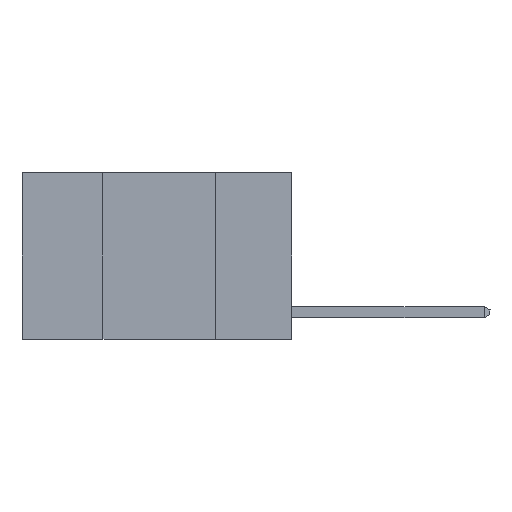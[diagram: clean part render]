
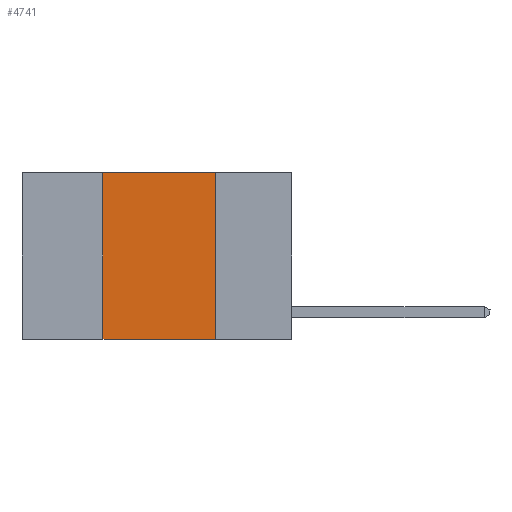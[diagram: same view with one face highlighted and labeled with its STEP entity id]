
A CAD part, left-side view. The second image highlights one B-rep face of the part: STEP entity #4741.
In plain terms, the highlighted planar face has unit normal (-1, 0, 0).
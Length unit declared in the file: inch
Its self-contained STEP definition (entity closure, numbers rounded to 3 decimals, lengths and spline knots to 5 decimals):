
#99 = FACE_OUTER_BOUND ( 'NONE', #6273, .T. ) ;
#701 = LINE ( 'NONE', #2503, #13827 ) ;
#1141 = VERTEX_POINT ( 'NONE', #3644 ) ;
#2503 = CARTESIAN_POINT ( 'NONE',  ( 0., 0.17, 0. ) ) ;
#2911 = DIRECTION ( 'NONE',  ( 1., 0., 0. ) ) ;
#3143 = ORIENTED_EDGE ( 'NONE', *, *, #4018, .F. ) ;
#3644 = CARTESIAN_POINT ( 'NONE',  ( 0., 0.17, -0.37 ) ) ;
#4018 = EDGE_CURVE ( 'NONE', #9808, #6234, #17129, .T. ) ;
#4741 = ADVANCED_FACE ( 'NONE', ( #99 ), #13741, .F. ) ;
#5187 = DIRECTION ( 'NONE',  ( 0., -1., 0. ) ) ;
#5517 = DIRECTION ( 'NONE',  ( 0., 0., -1. ) ) ;
#5796 = CARTESIAN_POINT ( 'NONE',  ( 0., 0.6, -0.37 ) ) ;
#5877 = ORIENTED_EDGE ( 'NONE', *, *, #19534, .T. ) ;
#6234 = VERTEX_POINT ( 'NONE', #14365 ) ;
#6273 = EDGE_LOOP ( 'NONE', ( #17300, #3143, #19536, #5877 ) ) ;
#7920 = CARTESIAN_POINT ( 'NONE',  ( 0., 0.42, 0. ) ) ;
#8238 = VECTOR ( 'NONE', #18033, 39.37008 ) ;
#8359 = EDGE_CURVE ( 'NONE', #10522, #9808, #13824, .T. ) ;
#8941 = DIRECTION ( 'NONE',  ( 0., 0., -1. ) ) ;
#9808 = VERTEX_POINT ( 'NONE', #14621 ) ;
#10199 = LINE ( 'NONE', #5796, #8238 ) ;
#10522 = VERTEX_POINT ( 'NONE', #15298 ) ;
#10896 = CARTESIAN_POINT ( 'NONE',  ( 0., 0.6, 0. ) ) ;
#12058 = AXIS2_PLACEMENT_3D ( 'NONE', #12228, #2911, #8941 ) ;
#12228 = CARTESIAN_POINT ( 'NONE',  ( 0., 0.6, 0. ) ) ;
#12716 = DIRECTION ( 'NONE',  ( 0., 0., 1. ) ) ;
#13741 = PLANE ( 'NONE',  #12058 ) ;
#13824 = LINE ( 'NONE', #7920, #15321 ) ;
#13827 = VECTOR ( 'NONE', #5517, 39.37008 ) ;
#14247 = VECTOR ( 'NONE', #5187, 39.37008 ) ;
#14365 = CARTESIAN_POINT ( 'NONE',  ( 0., 0.17, 0. ) ) ;
#14621 = CARTESIAN_POINT ( 'NONE',  ( 0., 0.42, 0. ) ) ;
#14649 = EDGE_CURVE ( 'NONE', #6234, #1141, #701, .T. ) ;
#15298 = CARTESIAN_POINT ( 'NONE',  ( 0., 0.42, -0.37 ) ) ;
#15321 = VECTOR ( 'NONE', #12716, 39.37008 ) ;
#17129 = LINE ( 'NONE', #10896, #14247 ) ;
#17300 = ORIENTED_EDGE ( 'NONE', *, *, #14649, .F. ) ;
#18033 = DIRECTION ( 'NONE',  ( 0., -1., 0. ) ) ;
#19534 = EDGE_CURVE ( 'NONE', #10522, #1141, #10199, .T. ) ;
#19536 = ORIENTED_EDGE ( 'NONE', *, *, #8359, .F. ) ;
